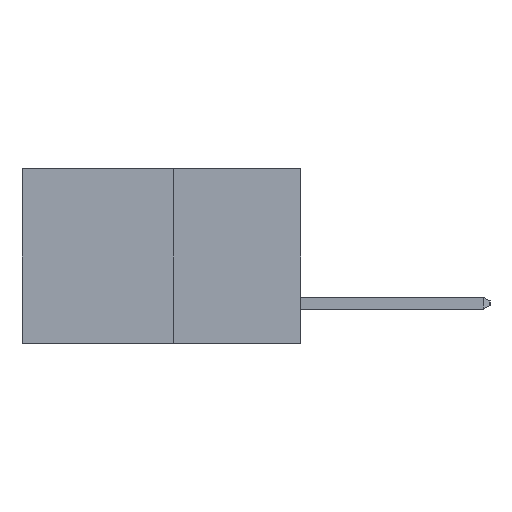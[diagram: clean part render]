
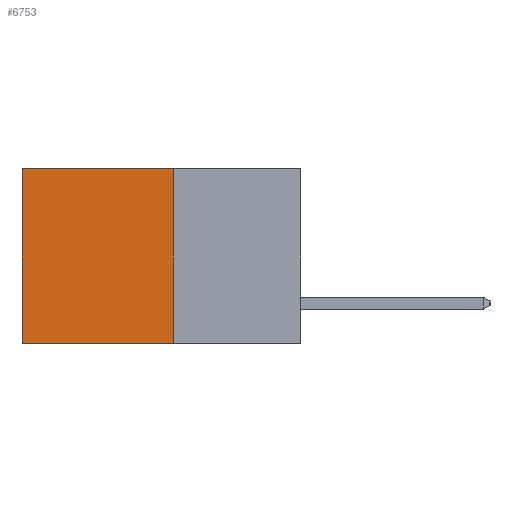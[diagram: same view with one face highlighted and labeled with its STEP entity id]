
A CAD part, left-side view. The second image highlights one B-rep face of the part: STEP entity #6753.
In plain terms, the highlighted planar face has unit normal (-1, 0, 0).
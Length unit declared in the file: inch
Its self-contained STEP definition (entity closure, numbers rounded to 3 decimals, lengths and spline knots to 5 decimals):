
#16 = LINE ( 'NONE', #2250, #5916 ) ;
#119 = DIRECTION ( 'NONE',  ( 1., 0., 0. ) ) ;
#891 = VERTEX_POINT ( 'NONE', #4364 ) ;
#2091 = VERTEX_POINT ( 'NONE', #6912 ) ;
#2096 = LINE ( 'NONE', #3782, #10791 ) ;
#2250 = CARTESIAN_POINT ( 'NONE',  ( 0.277, 0.27, -0.37 ) ) ;
#2416 = EDGE_CURVE ( 'NONE', #4554, #891, #13544, .T. ) ;
#3356 = ORIENTED_EDGE ( 'NONE', *, *, #2416, .T. ) ;
#3422 = FACE_OUTER_BOUND ( 'NONE', #7264, .T. ) ;
#3706 = PLANE ( 'NONE',  #9765 ) ;
#3782 = CARTESIAN_POINT ( 'NONE',  ( 0.277, 0.59, -0.37 ) ) ;
#3918 = CARTESIAN_POINT ( 'NONE',  ( 0.277, 0.27, 0. ) ) ;
#4196 = CARTESIAN_POINT ( 'NONE',  ( 0.277, 0.27, -0.37 ) ) ;
#4364 = CARTESIAN_POINT ( 'NONE',  ( 0.277, 0.59, 0. ) ) ;
#4448 = ORIENTED_EDGE ( 'NONE', *, *, #7884, .F. ) ;
#4554 = VERTEX_POINT ( 'NONE', #3918 ) ;
#5118 = LINE ( 'NONE', #14406, #13475 ) ;
#5427 = DIRECTION ( 'NONE',  ( 0., 0., -1. ) ) ;
#5916 = VECTOR ( 'NONE', #5427, 39.37008 ) ;
#6655 = EDGE_CURVE ( 'NONE', #891, #2091, #2096, .T. ) ;
#6753 = ADVANCED_FACE ( 'NONE', ( #3422 ), #3706, .F. ) ;
#6912 = CARTESIAN_POINT ( 'NONE',  ( 0.277, 0.59, -0.37 ) ) ;
#7023 = EDGE_CURVE ( 'NONE', #4554, #11717, #16, .T. ) ;
#7194 = DIRECTION ( 'NONE',  ( 0., 0., -1. ) ) ;
#7264 = EDGE_LOOP ( 'NONE', ( #11131, #4448, #9118, #3356 ) ) ;
#7884 = EDGE_CURVE ( 'NONE', #11717, #2091, #5118, .T. ) ;
#9118 = ORIENTED_EDGE ( 'NONE', *, *, #7023, .F. ) ;
#9765 = AXIS2_PLACEMENT_3D ( 'NONE', #4196, #119, #10117 ) ;
#10117 = DIRECTION ( 'NONE',  ( 0., 0., -1. ) ) ;
#10742 = VECTOR ( 'NONE', #14476, 39.37008 ) ;
#10791 = VECTOR ( 'NONE', #7194, 39.37008 ) ;
#10831 = CARTESIAN_POINT ( 'NONE',  ( 0.277, 0.27, -0.37 ) ) ;
#11131 = ORIENTED_EDGE ( 'NONE', *, *, #6655, .T. ) ;
#11717 = VERTEX_POINT ( 'NONE', #10831 ) ;
#12217 = CARTESIAN_POINT ( 'NONE',  ( 0.277, 0.27, 0. ) ) ;
#13475 = VECTOR ( 'NONE', #14203, 39.37008 ) ;
#13544 = LINE ( 'NONE', #12217, #10742 ) ;
#14203 = DIRECTION ( 'NONE',  ( 0., 1., 0. ) ) ;
#14406 = CARTESIAN_POINT ( 'NONE',  ( 0.277, 0.27, -0.37 ) ) ;
#14476 = DIRECTION ( 'NONE',  ( 0., 1., 0. ) ) ;
